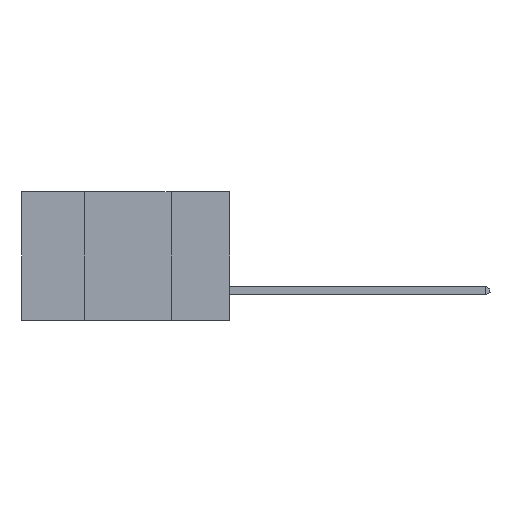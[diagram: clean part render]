
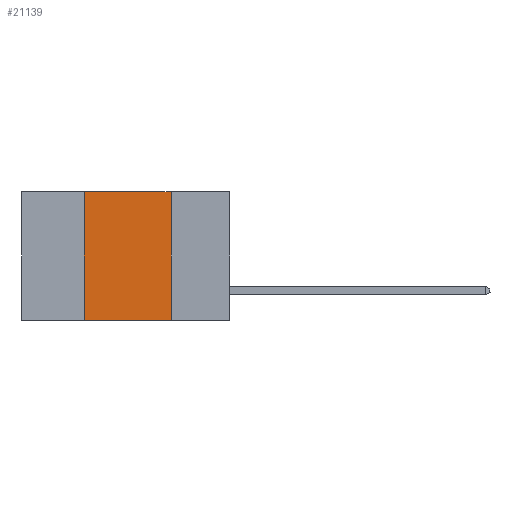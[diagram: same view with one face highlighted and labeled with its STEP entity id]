
A CAD part, left-side view. The second image highlights one B-rep face of the part: STEP entity #21139.
In plain terms, the highlighted planar face has unit normal (-1, 0, 0).
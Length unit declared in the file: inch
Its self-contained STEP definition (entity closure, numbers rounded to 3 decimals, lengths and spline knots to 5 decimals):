
#106 = CARTESIAN_POINT ( 'NONE',  ( 0., 0.6, 0. ) ) ;
#1346 = ORIENTED_EDGE ( 'NONE', *, *, #17628, .F. ) ;
#1765 = ORIENTED_EDGE ( 'NONE', *, *, #8034, .T. ) ;
#2012 = CARTESIAN_POINT ( 'NONE',  ( 0., 0.42, 0. ) ) ;
#2351 = VERTEX_POINT ( 'NONE', #17531 ) ;
#2685 = VECTOR ( 'NONE', #29202, 39.37008 ) ;
#2689 = CARTESIAN_POINT ( 'NONE',  ( 0., 0.17, 0. ) ) ;
#3419 = VECTOR ( 'NONE', #18226, 39.37008 ) ;
#4521 = DIRECTION ( 'NONE',  ( 0., -1., 0. ) ) ;
#4589 = DIRECTION ( 'NONE',  ( 1., 0., 0. ) ) ;
#5183 = VERTEX_POINT ( 'NONE', #20690 ) ;
#6563 = LINE ( 'NONE', #24603, #2685 ) ;
#7051 = LINE ( 'NONE', #2012, #12792 ) ;
#8034 = EDGE_CURVE ( 'NONE', #2351, #18613, #30424, .T. ) ;
#8112 = AXIS2_PLACEMENT_3D ( 'NONE', #106, #4589, #14478 ) ;
#10507 = ORIENTED_EDGE ( 'NONE', *, *, #11221, .F. ) ;
#11221 = EDGE_CURVE ( 'NONE', #2351, #5183, #7051, .T. ) ;
#12200 = PLANE ( 'NONE',  #8112 ) ;
#12792 = VECTOR ( 'NONE', #16695, 39.37008 ) ;
#14478 = DIRECTION ( 'NONE',  ( 0., 0., -1. ) ) ;
#15147 = CARTESIAN_POINT ( 'NONE',  ( 0., 0.6, -0.37 ) ) ;
#16695 = DIRECTION ( 'NONE',  ( 0., 0., 1. ) ) ;
#17531 = CARTESIAN_POINT ( 'NONE',  ( 0., 0.42, -0.37 ) ) ;
#17628 = EDGE_CURVE ( 'NONE', #21970, #18613, #6563, .T. ) ;
#18226 = DIRECTION ( 'NONE',  ( 0., -1., 0. ) ) ;
#18613 = VERTEX_POINT ( 'NONE', #27260 ) ;
#20047 = VECTOR ( 'NONE', #4521, 39.37008 ) ;
#20690 = CARTESIAN_POINT ( 'NONE',  ( 0., 0.42, 0. ) ) ;
#21139 = ADVANCED_FACE ( 'NONE', ( #27092 ), #12200, .F. ) ;
#21295 = CARTESIAN_POINT ( 'NONE',  ( 0., 0.6, 0. ) ) ;
#21970 = VERTEX_POINT ( 'NONE', #2689 ) ;
#22264 = EDGE_CURVE ( 'NONE', #5183, #21970, #26604, .T. ) ;
#24603 = CARTESIAN_POINT ( 'NONE',  ( 0., 0.17, 0. ) ) ;
#25028 = ORIENTED_EDGE ( 'NONE', *, *, #22264, .F. ) ;
#26604 = LINE ( 'NONE', #21295, #20047 ) ;
#27092 = FACE_OUTER_BOUND ( 'NONE', #30324, .T. ) ;
#27260 = CARTESIAN_POINT ( 'NONE',  ( 0., 0.17, -0.37 ) ) ;
#29202 = DIRECTION ( 'NONE',  ( 0., 0., -1. ) ) ;
#30324 = EDGE_LOOP ( 'NONE', ( #1346, #25028, #10507, #1765 ) ) ;
#30424 = LINE ( 'NONE', #15147, #3419 ) ;
